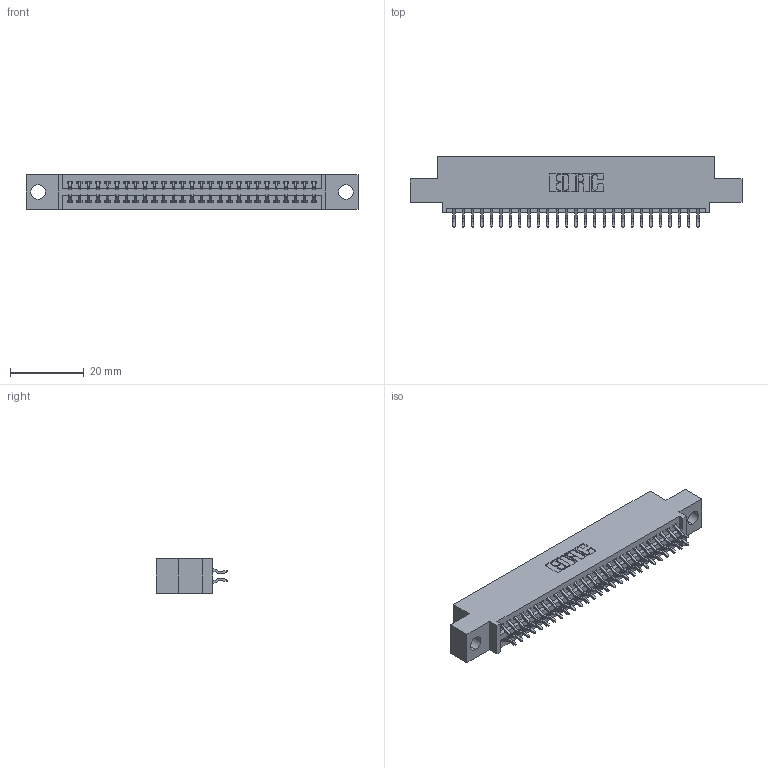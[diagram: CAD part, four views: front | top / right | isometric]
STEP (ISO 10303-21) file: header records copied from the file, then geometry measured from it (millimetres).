
FILE_DESCRIPTION (( 'STEP AP203' ), '1' );
FILE_NAME ('395-054-556-504.STEP', '2021-06-17T00:52:37', ( '' ), ( '' ), 'SwSTEP 2.0', 'SolidWorks 2020', '' );
FILE_SCHEMA (( 'CONFIG_CONTROL_DESIGN' ));
Length unit declared in the file: inch
Products named in the file (3): 395-054-556-504; 345 Part_0.110 Offset - 0.156 Dia-TI; 345-292-001_556 Tail
Assembly tree (55 placements, depth 2):
  395-054-556-504
    345 Part_0.110 Offset - 0.156 Dia-TI
    345-292-001_556 Tail  x54
Bounding box: 89.79 x 19.24 x 9.4 mm (x, y, z)
Volume: 8401.5 mm3; surface area: 12025.5 mm2
Topology: 55 solids, 55 shells, 3168 faces, 9407 edges, 6198 vertices
Faces by surface type: plane 2096, cylinder 1072
Entity records: 23975 total; most frequent: CARTESIAN_POINT 4054, ORIENTED_EDGE 3974, DIRECTION 3579, EDGE_CURVE 1987, VECTOR 1739, LINE 1739, VERTEX_POINT 1322, AXIS2_PLACEMENT_3D 920
